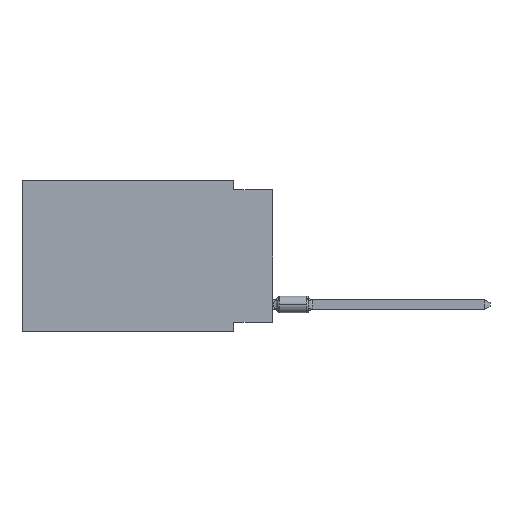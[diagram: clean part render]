
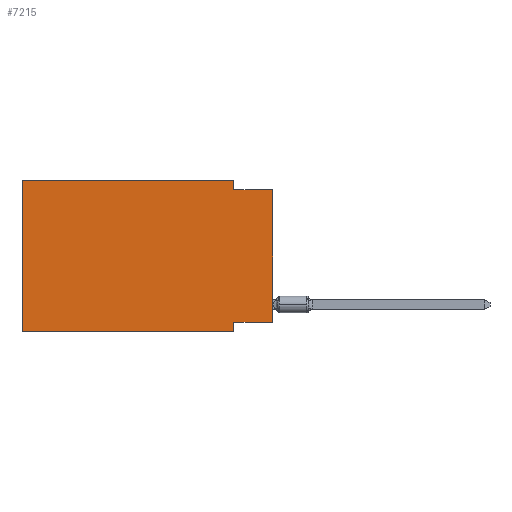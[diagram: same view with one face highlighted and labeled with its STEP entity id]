
A CAD part, left-side view. The second image highlights one B-rep face of the part: STEP entity #7215.
In plain terms, the highlighted planar face has unit normal (-1, 0, 0).
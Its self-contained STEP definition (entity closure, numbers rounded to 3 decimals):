
#145 = AXIS2_PLACEMENT_3D ( 'NONE', #11884, #9660, #6519 ) ;
#205 = LINE ( 'NONE', #2145, #12205 ) ;
#436 = ORIENTED_EDGE ( 'NONE', *, *, #5138, .F. ) ;
#453 = CARTESIAN_POINT ( 'NONE',  ( 0., 0., -9.271 ) ) ;
#481 = VERTEX_POINT ( 'NONE', #5945 ) ;
#829 = VECTOR ( 'NONE', #7764, 1000. ) ;
#941 = FACE_OUTER_BOUND ( 'NONE', #11076, .T. ) ;
#1067 = DIRECTION ( 'NONE',  ( 0., 0., -1. ) ) ;
#1215 = ORIENTED_EDGE ( 'NONE', *, *, #6023, .F. ) ;
#1614 = VECTOR ( 'NONE', #10586, 1000. ) ;
#1622 = CARTESIAN_POINT ( 'NONE',  ( 0., 0., -0.635 ) ) ;
#2145 = CARTESIAN_POINT ( 'NONE',  ( 0., 2.54, 0. ) ) ;
#2359 = EDGE_CURVE ( 'NONE', #3075, #481, #9441, .T. ) ;
#2937 = CARTESIAN_POINT ( 'NONE',  ( 0., 16.383, -9.906 ) ) ;
#3066 = ORIENTED_EDGE ( 'NONE', *, *, #7682, .T. ) ;
#3075 = VERTEX_POINT ( 'NONE', #6988 ) ;
#3353 = VECTOR ( 'NONE', #7163, 1000. ) ;
#3374 = CARTESIAN_POINT ( 'NONE',  ( 0., 0., -9.271 ) ) ;
#3417 = CARTESIAN_POINT ( 'NONE',  ( 0., 0., -0.635 ) ) ;
#3419 = LINE ( 'NONE', #6411, #9535 ) ;
#3420 = ORIENTED_EDGE ( 'NONE', *, *, #11166, .F. ) ;
#3876 = CARTESIAN_POINT ( 'NONE',  ( 0., 2.54, -9.906 ) ) ;
#4262 = DIRECTION ( 'NONE',  ( 0., -1., 0. ) ) ;
#4615 = EDGE_CURVE ( 'NONE', #4747, #3075, #9376, .T. ) ;
#4747 = VERTEX_POINT ( 'NONE', #2937 ) ;
#5138 = EDGE_CURVE ( 'NONE', #8257, #6689, #7548, .T. ) ;
#5180 = LINE ( 'NONE', #9337, #5586 ) ;
#5586 = VECTOR ( 'NONE', #8332, 1000. ) ;
#5945 = CARTESIAN_POINT ( 'NONE',  ( 0., 2.54, 0. ) ) ;
#6023 = EDGE_CURVE ( 'NONE', #12896, #8542, #11023, .T. ) ;
#6411 = CARTESIAN_POINT ( 'NONE',  ( 0., 16.383, -9.906 ) ) ;
#6519 = DIRECTION ( 'NONE',  ( 0., 0., -1. ) ) ;
#6520 = ORIENTED_EDGE ( 'NONE', *, *, #4615, .F. ) ;
#6689 = VERTEX_POINT ( 'NONE', #1622 ) ;
#6988 = CARTESIAN_POINT ( 'NONE',  ( 0., 16.383, 0. ) ) ;
#7163 = DIRECTION ( 'NONE',  ( 0., 0., 1. ) ) ;
#7182 = VECTOR ( 'NONE', #7716, 1000. ) ;
#7215 = ADVANCED_FACE ( 'NONE', ( #941 ), #9584, .F. ) ;
#7548 = LINE ( 'NONE', #3417, #829 ) ;
#7682 = EDGE_CURVE ( 'NONE', #4747, #10011, #3419, .T. ) ;
#7716 = DIRECTION ( 'NONE',  ( 0., 0., 1. ) ) ;
#7764 = DIRECTION ( 'NONE',  ( 0., -1., 0. ) ) ;
#7953 = EDGE_CURVE ( 'NONE', #8542, #10011, #5180, .T. ) ;
#8257 = VERTEX_POINT ( 'NONE', #13491 ) ;
#8332 = DIRECTION ( 'NONE',  ( 0., 0., -1. ) ) ;
#8409 = EDGE_CURVE ( 'NONE', #12896, #6689, #8723, .T. ) ;
#8542 = VERTEX_POINT ( 'NONE', #9284 ) ;
#8723 = LINE ( 'NONE', #8796, #7182 ) ;
#8796 = CARTESIAN_POINT ( 'NONE',  ( 0., 0., 0. ) ) ;
#9284 = CARTESIAN_POINT ( 'NONE',  ( 0., 2.54, -9.271 ) ) ;
#9310 = CARTESIAN_POINT ( 'NONE',  ( 0., 16.383, 0. ) ) ;
#9337 = CARTESIAN_POINT ( 'NONE',  ( 0., 2.54, -9.906 ) ) ;
#9376 = LINE ( 'NONE', #9310, #3353 ) ;
#9441 = LINE ( 'NONE', #11727, #1614 ) ;
#9534 = ORIENTED_EDGE ( 'NONE', *, *, #7953, .F. ) ;
#9535 = VECTOR ( 'NONE', #4262, 1000. ) ;
#9584 = PLANE ( 'NONE',  #145 ) ;
#9660 = DIRECTION ( 'NONE',  ( 1., 0., 0. ) ) ;
#10011 = VERTEX_POINT ( 'NONE', #3876 ) ;
#10013 = DIRECTION ( 'NONE',  ( 0., 1., 0. ) ) ;
#10586 = DIRECTION ( 'NONE',  ( 0., -1., 0. ) ) ;
#11023 = LINE ( 'NONE', #3374, #12089 ) ;
#11076 = EDGE_LOOP ( 'NONE', ( #13094, #436, #3420, #13830, #6520, #3066, #9534, #1215 ) ) ;
#11166 = EDGE_CURVE ( 'NONE', #481, #8257, #205, .T. ) ;
#11727 = CARTESIAN_POINT ( 'NONE',  ( 0., 16.383, 0. ) ) ;
#11884 = CARTESIAN_POINT ( 'NONE',  ( 0., 16.383, 0. ) ) ;
#12089 = VECTOR ( 'NONE', #10013, 1000. ) ;
#12205 = VECTOR ( 'NONE', #1067, 1000. ) ;
#12896 = VERTEX_POINT ( 'NONE', #453 ) ;
#13094 = ORIENTED_EDGE ( 'NONE', *, *, #8409, .T. ) ;
#13491 = CARTESIAN_POINT ( 'NONE',  ( 0., 2.54, -0.635 ) ) ;
#13830 = ORIENTED_EDGE ( 'NONE', *, *, #2359, .F. ) ;
